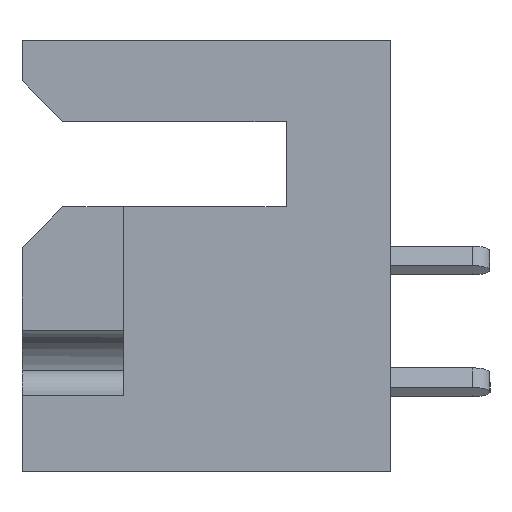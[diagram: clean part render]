
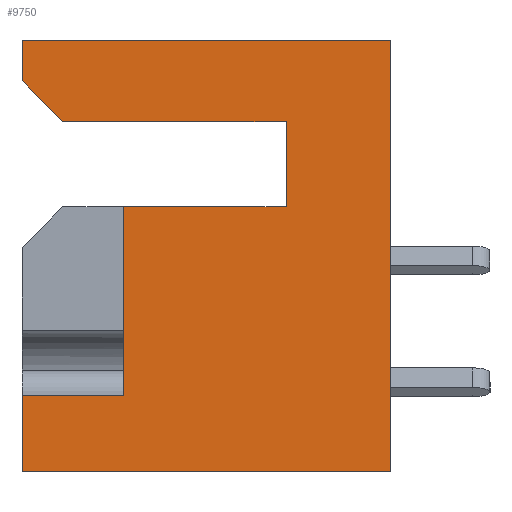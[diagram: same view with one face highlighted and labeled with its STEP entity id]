
A CAD part, left-side view. The second image highlights one B-rep face of the part: STEP entity #9750.
In plain terms, the highlighted planar face has unit normal (-1, 0, 0).
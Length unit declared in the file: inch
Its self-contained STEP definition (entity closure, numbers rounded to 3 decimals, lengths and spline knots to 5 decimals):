
#13 = ORIENTED_EDGE ( 'NONE', *, *, #11773, .T. ) ;
#350 = CARTESIAN_POINT ( 'NONE',  ( 0., 0.328, -0.437 ) ) ;
#696 = CARTESIAN_POINT ( 'NONE',  ( 0., 0.128, -0.205 ) ) ;
#702 = DIRECTION ( 'NONE',  ( 0., -1., 0. ) ) ;
#784 = LINE ( 'NONE', #696, #14022 ) ;
#804 = DIRECTION ( 'NONE',  ( 0., -1., 0. ) ) ;
#808 = LINE ( 'NONE', #4624, #5480 ) ;
#1495 = LINE ( 'NONE', #6477, #4240 ) ;
#1646 = EDGE_CURVE ( 'NONE', #4927, #13446, #11916, .T. ) ;
#1760 = CARTESIAN_POINT ( 'NONE',  ( 0., 0.453, -0.05 ) ) ;
#1772 = CARTESIAN_POINT ( 'NONE',  ( 0., 0.453, -0.437 ) ) ;
#1961 = EDGE_CURVE ( 'NONE', #6368, #4367, #7853, .T. ) ;
#1980 = CARTESIAN_POINT ( 'NONE',  ( 0., 0.453, 0. ) ) ;
#2222 = VECTOR ( 'NONE', #804, 39.37008 ) ;
#2237 = VERTEX_POINT ( 'NONE', #350 ) ;
#2353 = EDGE_CURVE ( 'NONE', #13812, #17033, #808, .T. ) ;
#2460 = ORIENTED_EDGE ( 'NONE', *, *, #1961, .T. ) ;
#2643 = AXIS2_PLACEMENT_3D ( 'NONE', #6030, #14407, #3226 ) ;
#2686 = VECTOR ( 'NONE', #15956, 39.37008 ) ;
#3057 = EDGE_CURVE ( 'NONE', #2237, #11124, #3742, .T. ) ;
#3226 = DIRECTION ( 'NONE',  ( 0., 0., -1. ) ) ;
#3742 = LINE ( 'NONE', #14739, #2686 ) ;
#3797 = LINE ( 'NONE', #15451, #12332 ) ;
#4240 = VECTOR ( 'NONE', #16085, 39.37008 ) ;
#4367 = VERTEX_POINT ( 'NONE', #14346 ) ;
#4461 = LINE ( 'NONE', #14312, #6583 ) ;
#4624 = CARTESIAN_POINT ( 'NONE',  ( 0., 0.453, 0. ) ) ;
#4805 = ORIENTED_EDGE ( 'NONE', *, *, #10949, .F. ) ;
#4927 = VERTEX_POINT ( 'NONE', #10032 ) ;
#5150 = DIRECTION ( 'NONE',  ( 0., 1., 0. ) ) ;
#5231 = DIRECTION ( 'NONE',  ( 0., -0.707, -0.707 ) ) ;
#5480 = VECTOR ( 'NONE', #702, 39.37008 ) ;
#5581 = FACE_OUTER_BOUND ( 'NONE', #11856, .T. ) ;
#5614 = ORIENTED_EDGE ( 'NONE', *, *, #2353, .F. ) ;
#5642 = ORIENTED_EDGE ( 'NONE', *, *, #14874, .T. ) ;
#5684 = VERTEX_POINT ( 'NONE', #15541 ) ;
#6022 = DIRECTION ( 'NONE',  ( 0., 0., 1. ) ) ;
#6030 = CARTESIAN_POINT ( 'NONE',  ( 0., 0.453, 0. ) ) ;
#6185 = EDGE_CURVE ( 'NONE', #17446, #6309, #8918, .T. ) ;
#6309 = VERTEX_POINT ( 'NONE', #8724 ) ;
#6368 = VERTEX_POINT ( 'NONE', #1760 ) ;
#6405 = EDGE_CURVE ( 'NONE', #6309, #4367, #3797, .T. ) ;
#6477 = CARTESIAN_POINT ( 'NONE',  ( 0., 0., 0. ) ) ;
#6545 = CARTESIAN_POINT ( 'NONE',  ( 0., 0.128, -0.205 ) ) ;
#6564 = ORIENTED_EDGE ( 'NONE', *, *, #1646, .F. ) ;
#6583 = VECTOR ( 'NONE', #10414, 39.37008 ) ;
#7853 = LINE ( 'NONE', #9337, #16657 ) ;
#8651 = ORIENTED_EDGE ( 'NONE', *, *, #6185, .F. ) ;
#8695 = CARTESIAN_POINT ( 'NONE',  ( 0., 0.328, -0.437 ) ) ;
#8724 = CARTESIAN_POINT ( 'NONE',  ( 0., 0.128, -0.1 ) ) ;
#8918 = LINE ( 'NONE', #11175, #10423 ) ;
#8983 = ORIENTED_EDGE ( 'NONE', *, *, #15975, .T. ) ;
#9201 = ORIENTED_EDGE ( 'NONE', *, *, #6405, .F. ) ;
#9337 = CARTESIAN_POINT ( 'NONE',  ( 0., 0.403, -0.1 ) ) ;
#9750 = ADVANCED_FACE ( 'NONE', ( #5581 ), #14291, .F. ) ;
#10032 = CARTESIAN_POINT ( 'NONE',  ( 0., 0.453, -0.531 ) ) ;
#10051 = DIRECTION ( 'NONE',  ( 0., 0., 1. ) ) ;
#10414 = DIRECTION ( 'NONE',  ( 0., 0., 1. ) ) ;
#10423 = VECTOR ( 'NONE', #10051, 39.37008 ) ;
#10949 = EDGE_CURVE ( 'NONE', #6368, #13812, #4461, .T. ) ;
#11124 = VERTEX_POINT ( 'NONE', #13307 ) ;
#11175 = CARTESIAN_POINT ( 'NONE',  ( 0., 0.128, -0.1 ) ) ;
#11611 = CARTESIAN_POINT ( 'NONE',  ( 0., 0.453, -0.531 ) ) ;
#11773 = EDGE_CURVE ( 'NONE', #5684, #17033, #1495, .T. ) ;
#11856 = EDGE_LOOP ( 'NONE', ( #8983, #6564, #5642, #13, #5614, #4805, #2460, #9201, #8651, #13150, #17019 ) ) ;
#11916 = LINE ( 'NONE', #1980, #17740 ) ;
#12332 = VECTOR ( 'NONE', #16721, 39.37008 ) ;
#13150 = ORIENTED_EDGE ( 'NONE', *, *, #13645, .T. ) ;
#13307 = CARTESIAN_POINT ( 'NONE',  ( 0., 0.328, -0.205 ) ) ;
#13446 = VERTEX_POINT ( 'NONE', #1772 ) ;
#13542 = CARTESIAN_POINT ( 'NONE',  ( 0., 0.453, 0. ) ) ;
#13645 = EDGE_CURVE ( 'NONE', #17446, #11124, #784, .T. ) ;
#13812 = VERTEX_POINT ( 'NONE', #13542 ) ;
#13927 = VECTOR ( 'NONE', #15615, 39.37008 ) ;
#14022 = VECTOR ( 'NONE', #5150, 39.37008 ) ;
#14291 = PLANE ( 'NONE',  #2643 ) ;
#14312 = CARTESIAN_POINT ( 'NONE',  ( 0., 0.453, 0. ) ) ;
#14346 = CARTESIAN_POINT ( 'NONE',  ( 0., 0.403, -0.1 ) ) ;
#14407 = DIRECTION ( 'NONE',  ( 1., 0., 0. ) ) ;
#14739 = CARTESIAN_POINT ( 'NONE',  ( 0., 0.328, -0.205 ) ) ;
#14874 = EDGE_CURVE ( 'NONE', #4927, #5684, #17623, .T. ) ;
#15451 = CARTESIAN_POINT ( 'NONE',  ( 0., 0.128, -0.1 ) ) ;
#15541 = CARTESIAN_POINT ( 'NONE',  ( 0., 0., -0.531 ) ) ;
#15615 = DIRECTION ( 'NONE',  ( 0., 1., 0. ) ) ;
#15956 = DIRECTION ( 'NONE',  ( 0., 0., 1. ) ) ;
#15975 = EDGE_CURVE ( 'NONE', #2237, #13446, #17593, .T. ) ;
#16085 = DIRECTION ( 'NONE',  ( 0., 0., 1. ) ) ;
#16657 = VECTOR ( 'NONE', #5231, 39.37008 ) ;
#16721 = DIRECTION ( 'NONE',  ( 0., 1., 0. ) ) ;
#16722 = CARTESIAN_POINT ( 'NONE',  ( 0., 0., 0. ) ) ;
#17019 = ORIENTED_EDGE ( 'NONE', *, *, #3057, .F. ) ;
#17033 = VERTEX_POINT ( 'NONE', #16722 ) ;
#17446 = VERTEX_POINT ( 'NONE', #6545 ) ;
#17593 = LINE ( 'NONE', #8695, #13927 ) ;
#17623 = LINE ( 'NONE', #11611, #2222 ) ;
#17740 = VECTOR ( 'NONE', #6022, 39.37008 ) ;
